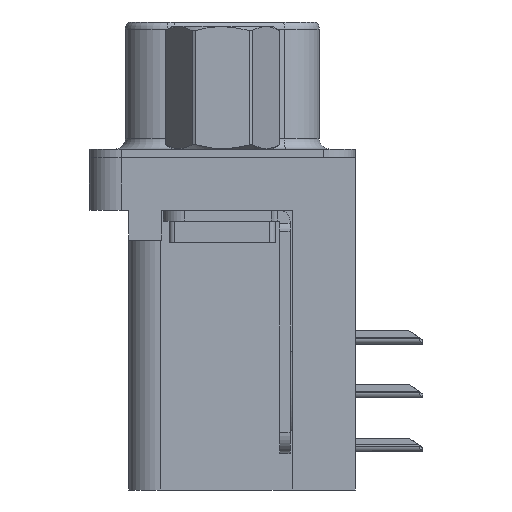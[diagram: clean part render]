
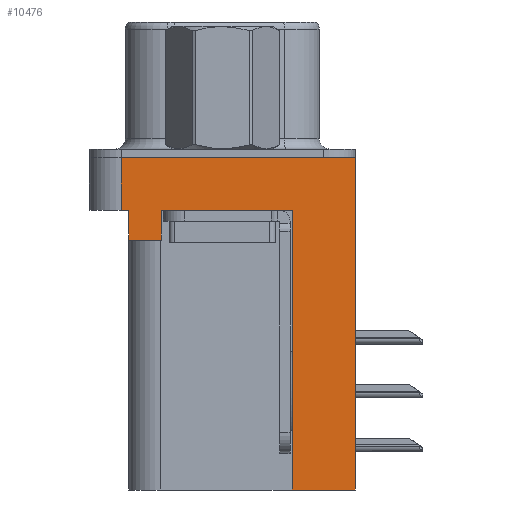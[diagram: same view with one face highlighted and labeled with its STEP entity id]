
A CAD part, left-side view. The second image highlights one B-rep face of the part: STEP entity #10476.
In plain terms, the highlighted planar face has unit normal (-1, 0, 0).
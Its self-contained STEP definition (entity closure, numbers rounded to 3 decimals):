
#130 = VECTOR ( 'NONE', #37273, 1000. ) ;
#163 = CARTESIAN_POINT ( 'NONE',  ( -2.91, -6.275, -2.5 ) ) ;
#872 = DIRECTION ( 'NONE',  ( -1., 0., 0. ) ) ;
#1032 = EDGE_CURVE ( 'NONE', #24898, #12191, #33099, .T. ) ;
#1211 = EDGE_CURVE ( 'NONE', #17299, #12191, #18548, .T. ) ;
#2265 = CARTESIAN_POINT ( 'NONE',  ( -2.91, 2.895, -3.9 ) ) ;
#3020 = LINE ( 'NONE', #35493, #11444 ) ;
#3365 = DIRECTION ( 'NONE',  ( 0., -1., 0. ) ) ;
#5058 = CARTESIAN_POINT ( 'NONE',  ( -2.91, -3.295, -15.7 ) ) ;
#5317 = LINE ( 'NONE', #38861, #21288 ) ;
#5345 = EDGE_LOOP ( 'NONE', ( #20975, #21538, #29016, #19290, #9781, #25501, #11533, #22767, #37428, #35906 ) ) ;
#5888 = AXIS2_PLACEMENT_3D ( 'NONE', #19940, #872, #23160 ) ;
#6340 = LINE ( 'NONE', #28508, #39408 ) ;
#7270 = EDGE_CURVE ( 'NONE', #39333, #24898, #3020, .T. ) ;
#7574 = DIRECTION ( 'NONE',  ( 0., 0., 1. ) ) ;
#8107 = DIRECTION ( 'NONE',  ( 0., -1., 0. ) ) ;
#9781 = ORIENTED_EDGE ( 'NONE', *, *, #7270, .F. ) ;
#10064 = EDGE_CURVE ( 'NONE', #22065, #17000, #29252, .T. ) ;
#10476 = ADVANCED_FACE ( 'NONE', ( #40700 ), #16748, .T. ) ;
#11444 = VECTOR ( 'NONE', #28967, 1000. ) ;
#11533 = ORIENTED_EDGE ( 'NONE', *, *, #24001, .T. ) ;
#11559 = CARTESIAN_POINT ( 'NONE',  ( -2.91, 4.775, 0. ) ) ;
#11790 = CARTESIAN_POINT ( 'NONE',  ( -2.91, -6.275, 0. ) ) ;
#12191 = VERTEX_POINT ( 'NONE', #22017 ) ;
#12286 = VECTOR ( 'NONE', #14678, 1000. ) ;
#12887 = CARTESIAN_POINT ( 'NONE',  ( -2.91, 2.895, -3.9 ) ) ;
#14299 = VECTOR ( 'NONE', #7574, 1000. ) ;
#14678 = DIRECTION ( 'NONE',  ( 0., 0., 1. ) ) ;
#15038 = CARTESIAN_POINT ( 'NONE',  ( -2.91, 4.425, -3.9 ) ) ;
#15255 = EDGE_CURVE ( 'NONE', #25746, #22065, #6340, .T. ) ;
#16748 = PLANE ( 'NONE',  #5888 ) ;
#17000 = VERTEX_POINT ( 'NONE', #20835 ) ;
#17299 = VERTEX_POINT ( 'NONE', #18979 ) ;
#17530 = VECTOR ( 'NONE', #8107, 1000. ) ;
#18548 = LINE ( 'NONE', #30298, #17530 ) ;
#18979 = CARTESIAN_POINT ( 'NONE',  ( -2.91, 4.775, -2.5 ) ) ;
#19290 = ORIENTED_EDGE ( 'NONE', *, *, #1032, .F. ) ;
#19940 = CARTESIAN_POINT ( 'NONE',  ( -2.91, -6.275, -2.5 ) ) ;
#19971 = VERTEX_POINT ( 'NONE', #11790 ) ;
#20543 = VERTEX_POINT ( 'NONE', #11559 ) ;
#20835 = CARTESIAN_POINT ( 'NONE',  ( -2.91, -3.295, -2.5 ) ) ;
#20975 = ORIENTED_EDGE ( 'NONE', *, *, #22184, .F. ) ;
#20982 = CARTESIAN_POINT ( 'NONE',  ( -2.91, 2.895, -2.5 ) ) ;
#21288 = VECTOR ( 'NONE', #22844, 1000. ) ;
#21357 = DIRECTION ( 'NONE',  ( 0., 0., 1. ) ) ;
#21538 = ORIENTED_EDGE ( 'NONE', *, *, #39548, .F. ) ;
#21551 = VECTOR ( 'NONE', #21357, 1000. ) ;
#22017 = CARTESIAN_POINT ( 'NONE',  ( -2.91, 4.425, -2.5 ) ) ;
#22065 = VERTEX_POINT ( 'NONE', #34991 ) ;
#22184 = EDGE_CURVE ( 'NONE', #20543, #19971, #36488, .T. ) ;
#22552 = LINE ( 'NONE', #2265, #21551 ) ;
#22767 = ORIENTED_EDGE ( 'NONE', *, *, #10064, .F. ) ;
#22844 = DIRECTION ( 'NONE',  ( 0., 0., 1. ) ) ;
#23160 = DIRECTION ( 'NONE',  ( 0., 0., 1. ) ) ;
#24001 = EDGE_CURVE ( 'NONE', #37549, #17000, #28276, .T. ) ;
#24647 = EDGE_CURVE ( 'NONE', #25746, #19971, #5317, .T. ) ;
#24898 = VERTEX_POINT ( 'NONE', #15038 ) ;
#25303 = DIRECTION ( 'NONE',  ( 0., 1., 0. ) ) ;
#25501 = ORIENTED_EDGE ( 'NONE', *, *, #35129, .T. ) ;
#25746 = VERTEX_POINT ( 'NONE', #32820 ) ;
#27908 = VECTOR ( 'NONE', #38790, 1000. ) ;
#28276 = LINE ( 'NONE', #163, #35855 ) ;
#28508 = CARTESIAN_POINT ( 'NONE',  ( -2.91, -3.295, -15.7 ) ) ;
#28967 = DIRECTION ( 'NONE',  ( 0., 1., 0. ) ) ;
#29016 = ORIENTED_EDGE ( 'NONE', *, *, #1211, .T. ) ;
#29032 = CARTESIAN_POINT ( 'NONE',  ( -2.91, -6.275, 0. ) ) ;
#29252 = LINE ( 'NONE', #5058, #12286 ) ;
#30298 = CARTESIAN_POINT ( 'NONE',  ( -2.91, -6.275, -2.5 ) ) ;
#31685 = CARTESIAN_POINT ( 'NONE',  ( -2.91, 4.425, -3.9 ) ) ;
#32304 = LINE ( 'NONE', #33168, #14299 ) ;
#32820 = CARTESIAN_POINT ( 'NONE',  ( -2.91, -6.275, -15.7 ) ) ;
#33099 = LINE ( 'NONE', #31685, #130 ) ;
#33168 = CARTESIAN_POINT ( 'NONE',  ( -2.91, 4.775, -2.5 ) ) ;
#34991 = CARTESIAN_POINT ( 'NONE',  ( -2.91, -3.295, -15.7 ) ) ;
#35129 = EDGE_CURVE ( 'NONE', #39333, #37549, #22552, .T. ) ;
#35493 = CARTESIAN_POINT ( 'NONE',  ( -2.91, 4.425, -3.9 ) ) ;
#35855 = VECTOR ( 'NONE', #3365, 1000. ) ;
#35906 = ORIENTED_EDGE ( 'NONE', *, *, #24647, .T. ) ;
#36488 = LINE ( 'NONE', #29032, #27908 ) ;
#37273 = DIRECTION ( 'NONE',  ( 0., 0., 1. ) ) ;
#37428 = ORIENTED_EDGE ( 'NONE', *, *, #15255, .F. ) ;
#37549 = VERTEX_POINT ( 'NONE', #20982 ) ;
#38790 = DIRECTION ( 'NONE',  ( 0., -1., 0. ) ) ;
#38861 = CARTESIAN_POINT ( 'NONE',  ( -2.91, -6.275, -2.5 ) ) ;
#39333 = VERTEX_POINT ( 'NONE', #12887 ) ;
#39408 = VECTOR ( 'NONE', #25303, 1000. ) ;
#39548 = EDGE_CURVE ( 'NONE', #17299, #20543, #32304, .T. ) ;
#40700 = FACE_OUTER_BOUND ( 'NONE', #5345, .T. ) ;
